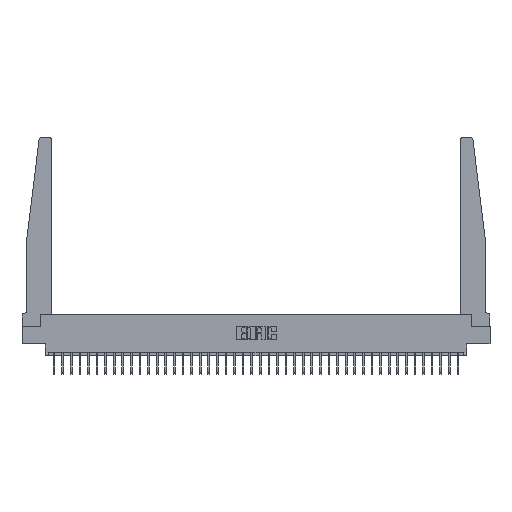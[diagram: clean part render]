
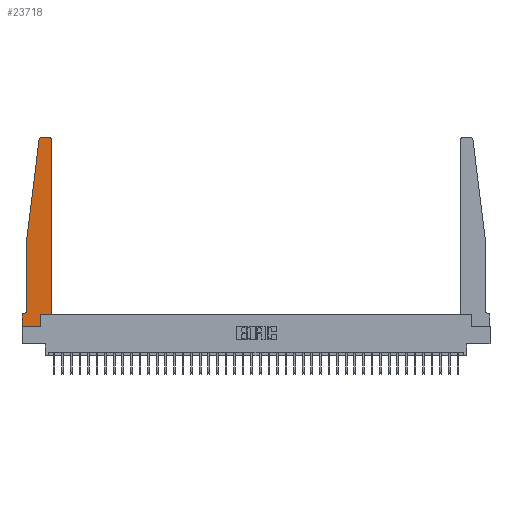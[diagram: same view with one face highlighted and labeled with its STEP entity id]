
A CAD part, top view. The second image highlights one B-rep face of the part: STEP entity #23718.
In plain terms, the highlighted planar face has unit normal (0, 0, 1).
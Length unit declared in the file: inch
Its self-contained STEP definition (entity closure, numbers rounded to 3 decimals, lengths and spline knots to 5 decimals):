
#206 = LINE ( 'NONE', #15494, #20328 ) ;
#923 = VECTOR ( 'NONE', #20582, 39.37008 ) ;
#993 = EDGE_CURVE ( 'NONE', #1062, #27929, #25249, .T. ) ;
#1062 = VERTEX_POINT ( 'NONE', #9648 ) ;
#1183 = LINE ( 'NONE', #17442, #29091 ) ;
#1733 = DIRECTION ( 'NONE',  ( 0., -1., 0. ) ) ;
#2065 = DIRECTION ( 'NONE',  ( -1., 0., 0. ) ) ;
#2295 = DIRECTION ( 'NONE',  ( 0., 0., 1. ) ) ;
#2414 = EDGE_CURVE ( 'NONE', #3167, #6264, #21854, .T. ) ;
#2559 = EDGE_CURVE ( 'NONE', #31799, #23253, #3753, .T. ) ;
#3167 = VERTEX_POINT ( 'NONE', #15611 ) ;
#3637 = VECTOR ( 'NONE', #12607, 39.37008 ) ;
#3753 = LINE ( 'NONE', #23771, #16923 ) ;
#4453 = EDGE_CURVE ( 'NONE', #8263, #1062, #1183, .T. ) ;
#4526 = DIRECTION ( 'NONE',  ( 0., 0., 1. ) ) ;
#4833 = CARTESIAN_POINT ( 'NONE',  ( 0.27653, 2.75, 0.37 ) ) ;
#5264 = CARTESIAN_POINT ( 'NONE',  ( 0.425, 0.18, 0.37 ) ) ;
#5638 = DIRECTION ( 'NONE',  ( -1., 0., 0. ) ) ;
#6264 = VERTEX_POINT ( 'NONE', #22487 ) ;
#6385 = ORIENTED_EDGE ( 'NONE', *, *, #23100, .T. ) ;
#6427 = AXIS2_PLACEMENT_3D ( 'NONE', #27636, #11924, #30275 ) ;
#6480 = VECTOR ( 'NONE', #5638, 39.37008 ) ;
#7093 = EDGE_CURVE ( 'NONE', #13277, #26546, #28540, .T. ) ;
#8071 = DIRECTION ( 'NONE',  ( 0., 1., 0. ) ) ;
#8263 = VERTEX_POINT ( 'NONE', #29774 ) ;
#8445 = ORIENTED_EDGE ( 'NONE', *, *, #4453, .T. ) ;
#8598 = CIRCLE ( 'NONE', #6427, 0.03 ) ;
#8838 = ORIENTED_EDGE ( 'NONE', *, *, #2414, .T. ) ;
#8877 = ORIENTED_EDGE ( 'NONE', *, *, #22950, .T. ) ;
#9300 = EDGE_CURVE ( 'NONE', #26546, #3167, #33769, .T. ) ;
#9648 = CARTESIAN_POINT ( 'NONE',  ( 0.065, 0.2375, 0.37 ) ) ;
#9706 = PLANE ( 'NONE',  #17407 ) ;
#9964 = CARTESIAN_POINT ( 'NONE',  ( 0.065, 1.25, 0.37 ) ) ;
#10079 = ORIENTED_EDGE ( 'NONE', *, *, #7093, .T. ) ;
#10865 = VECTOR ( 'NONE', #18354, 39.37008 ) ;
#11111 = CIRCLE ( 'NONE', #14212, 0.03 ) ;
#11580 = CARTESIAN_POINT ( 'NONE',  ( 0., 0.1875, 0.37 ) ) ;
#11924 = DIRECTION ( 'NONE',  ( 0., 0., 1. ) ) ;
#12558 = ORIENTED_EDGE ( 'NONE', *, *, #24066, .T. ) ;
#12607 = DIRECTION ( 'NONE',  ( -0.122, -0.992, 0. ) ) ;
#12945 = CARTESIAN_POINT ( 'NONE',  ( 0.395, 2.75, 0.37 ) ) ;
#13189 = DIRECTION ( 'NONE',  ( 1., 0., 0. ) ) ;
#13277 = VERTEX_POINT ( 'NONE', #11580 ) ;
#13514 = EDGE_CURVE ( 'NONE', #15381, #22543, #206, .T. ) ;
#13582 = EDGE_CURVE ( 'NONE', #6264, #31799, #31802, .T. ) ;
#13826 = CARTESIAN_POINT ( 'NONE',  ( 0.24675, 2.72367, 0.37 ) ) ;
#14212 = AXIS2_PLACEMENT_3D ( 'NONE', #18019, #2295, #20651 ) ;
#14419 = CARTESIAN_POINT ( 'NONE',  ( 0., 0., 0.37 ) ) ;
#14605 = VECTOR ( 'NONE', #32819, 39.37008 ) ;
#14968 = CARTESIAN_POINT ( 'NONE',  ( 0., 0.1875, 0.37 ) ) ;
#15376 = DIRECTION ( 'NONE',  ( -1., 0., 0. ) ) ;
#15381 = VERTEX_POINT ( 'NONE', #12945 ) ;
#15494 = CARTESIAN_POINT ( 'NONE',  ( 0.25, 2.75, 0.37 ) ) ;
#15611 = CARTESIAN_POINT ( 'NONE',  ( 0.2605, 0., 0.37 ) ) ;
#16923 = VECTOR ( 'NONE', #8071, 39.37008 ) ;
#17407 = AXIS2_PLACEMENT_3D ( 'NONE', #14968, #4526, #22879 ) ;
#17442 = CARTESIAN_POINT ( 'NONE',  ( 0.065, 1.25, 0.37 ) ) ;
#17617 = LINE ( 'NONE', #9964, #3637 ) ;
#17687 = EDGE_LOOP ( 'NONE', ( #31801, #21995, #6385, #8445, #27301, #12558, #10079, #19556, #8838, #24442, #28960, #8877 ) ) ;
#17958 = CARTESIAN_POINT ( 'NONE',  ( 0.2605, 0.18, 0.37 ) ) ;
#18019 = CARTESIAN_POINT ( 'NONE',  ( 0.27653, 2.72, 0.37 ) ) ;
#18354 = DIRECTION ( 'NONE',  ( 1., 0., 0. ) ) ;
#19509 = CARTESIAN_POINT ( 'NONE',  ( 0.015, 0.2375, 0.37 ) ) ;
#19556 = ORIENTED_EDGE ( 'NONE', *, *, #9300, .T. ) ;
#20328 = VECTOR ( 'NONE', #15376, 39.37008 ) ;
#20582 = DIRECTION ( 'NONE',  ( 0., 1., 0. ) ) ;
#20651 = DIRECTION ( 'NONE',  ( 1., 0., 0. ) ) ;
#21090 = CARTESIAN_POINT ( 'NONE',  ( 0.015, 0.1875, 0.37 ) ) ;
#21854 = LINE ( 'NONE', #17958, #923 ) ;
#21995 = ORIENTED_EDGE ( 'NONE', *, *, #27784, .T. ) ;
#22269 = CARTESIAN_POINT ( 'NONE',  ( 0., 0., 0.37 ) ) ;
#22487 = CARTESIAN_POINT ( 'NONE',  ( 0.2605, 0.18, 0.37 ) ) ;
#22543 = VERTEX_POINT ( 'NONE', #4833 ) ;
#22879 = DIRECTION ( 'NONE',  ( 1., 0., 0. ) ) ;
#22950 = EDGE_CURVE ( 'NONE', #23253, #15381, #8598, .T. ) ;
#23100 = EDGE_CURVE ( 'NONE', #28698, #8263, #17617, .T. ) ;
#23119 = DIRECTION ( 'NONE',  ( 0., 0., -1. ) ) ;
#23253 = VERTEX_POINT ( 'NONE', #28853 ) ;
#23718 = ADVANCED_FACE ( 'NONE', ( #31917 ), #9706, .T. ) ;
#23771 = CARTESIAN_POINT ( 'NONE',  ( 0.425, 0.18, 0.37 ) ) ;
#24066 = EDGE_CURVE ( 'NONE', #27929, #13277, #27393, .T. ) ;
#24442 = ORIENTED_EDGE ( 'NONE', *, *, #13582, .T. ) ;
#25249 = CIRCLE ( 'NONE', #28822, 0.05 ) ;
#26546 = VERTEX_POINT ( 'NONE', #14419 ) ;
#26648 = CARTESIAN_POINT ( 'NONE',  ( 0.065, 0.1875, 0.37 ) ) ;
#26843 = VECTOR ( 'NONE', #13189, 39.37008 ) ;
#27301 = ORIENTED_EDGE ( 'NONE', *, *, #993, .T. ) ;
#27393 = LINE ( 'NONE', #26648, #6480 ) ;
#27636 = CARTESIAN_POINT ( 'NONE',  ( 0.395, 2.72, 0.37 ) ) ;
#27784 = EDGE_CURVE ( 'NONE', #22543, #28698, #11111, .T. ) ;
#27929 = VERTEX_POINT ( 'NONE', #21090 ) ;
#27951 = CARTESIAN_POINT ( 'NONE',  ( 0.425, 0.18, 0.37 ) ) ;
#28540 = LINE ( 'NONE', #22269, #14605 ) ;
#28698 = VERTEX_POINT ( 'NONE', #13826 ) ;
#28822 = AXIS2_PLACEMENT_3D ( 'NONE', #19509, #23119, #2065 ) ;
#28853 = CARTESIAN_POINT ( 'NONE',  ( 0.425, 2.72, 0.37 ) ) ;
#28881 = CARTESIAN_POINT ( 'NONE',  ( 0., 0., 0.37 ) ) ;
#28960 = ORIENTED_EDGE ( 'NONE', *, *, #2559, .T. ) ;
#29091 = VECTOR ( 'NONE', #1733, 39.37008 ) ;
#29774 = CARTESIAN_POINT ( 'NONE',  ( 0.065, 1.25, 0.37 ) ) ;
#30275 = DIRECTION ( 'NONE',  ( 1., 0., 0. ) ) ;
#31799 = VERTEX_POINT ( 'NONE', #27951 ) ;
#31801 = ORIENTED_EDGE ( 'NONE', *, *, #13514, .T. ) ;
#31802 = LINE ( 'NONE', #5264, #10865 ) ;
#31917 = FACE_OUTER_BOUND ( 'NONE', #17687, .T. ) ;
#32819 = DIRECTION ( 'NONE',  ( 0., -1., 0. ) ) ;
#33769 = LINE ( 'NONE', #28881, #26843 ) ;
